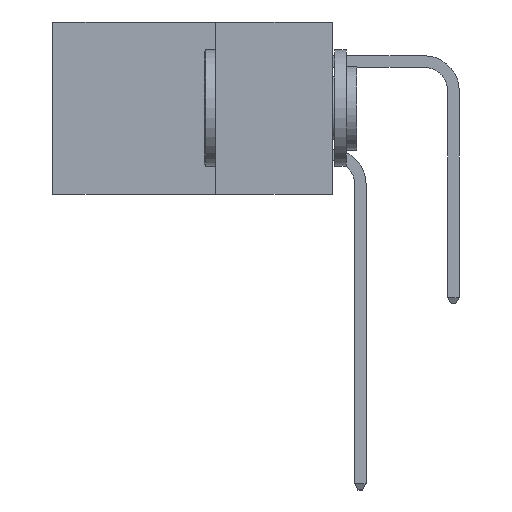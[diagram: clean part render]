
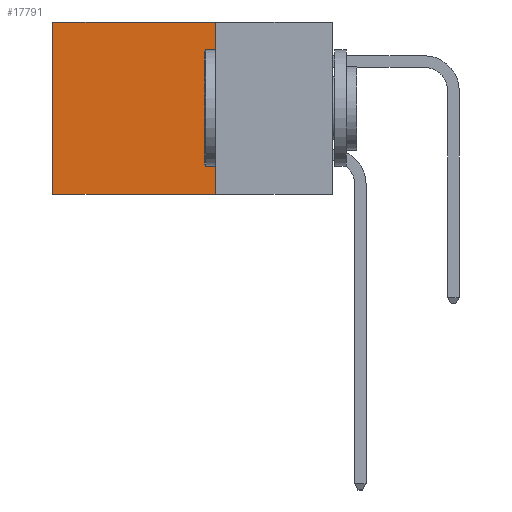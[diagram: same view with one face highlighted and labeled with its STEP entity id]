
A CAD part, left-side view. The second image highlights one B-rep face of the part: STEP entity #17791.
In plain terms, the highlighted planar face has unit normal (-1, 0, 0).
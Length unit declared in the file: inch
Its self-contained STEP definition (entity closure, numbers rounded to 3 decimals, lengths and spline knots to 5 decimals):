
#78 = EDGE_CURVE ( 'NONE', #25785, #3793, #5876, .T. ) ;
#630 = ORIENTED_EDGE ( 'NONE', *, *, #948, .F. ) ;
#640 = CARTESIAN_POINT ( 'NONE',  ( 0.2615, 0.25, -0.37 ) ) ;
#733 = DIRECTION ( 'NONE',  ( 0., 0., -1. ) ) ;
#948 = EDGE_CURVE ( 'NONE', #25785, #17775, #1451, .T. ) ;
#969 = CARTESIAN_POINT ( 'NONE',  ( 0.2615, 0.6, 0. ) ) ;
#1451 = LINE ( 'NONE', #21798, #7230 ) ;
#2162 = VERTEX_POINT ( 'NONE', #17096 ) ;
#3793 = VERTEX_POINT ( 'NONE', #969 ) ;
#5876 = LINE ( 'NONE', #25469, #10889 ) ;
#6764 = EDGE_CURVE ( 'NONE', #17775, #2162, #26233, .T. ) ;
#7230 = VECTOR ( 'NONE', #18867, 39.37008 ) ;
#8569 = EDGE_LOOP ( 'NONE', ( #27590, #21022, #630, #22609 ) ) ;
#9341 = PLANE ( 'NONE',  #25838 ) ;
#10278 = FACE_OUTER_BOUND ( 'NONE', #8569, .T. ) ;
#10849 = DIRECTION ( 'NONE',  ( 0., 1., 0. ) ) ;
#10889 = VECTOR ( 'NONE', #15597, 39.37008 ) ;
#13585 = DIRECTION ( 'NONE',  ( 1., 0., 0. ) ) ;
#14893 = VECTOR ( 'NONE', #10849, 39.37008 ) ;
#15597 = DIRECTION ( 'NONE',  ( 0., 1., 0. ) ) ;
#15653 = DIRECTION ( 'NONE',  ( 0., 0., -1. ) ) ;
#15832 = CARTESIAN_POINT ( 'NONE',  ( 0.2615, 0.25, 0. ) ) ;
#17096 = CARTESIAN_POINT ( 'NONE',  ( 0.2615, 0.6, -0.37 ) ) ;
#17204 = CARTESIAN_POINT ( 'NONE',  ( 0.2615, 0.25, -0.37 ) ) ;
#17261 = VECTOR ( 'NONE', #15653, 39.37008 ) ;
#17706 = CARTESIAN_POINT ( 'NONE',  ( 0.2615, 0.6, -0.37 ) ) ;
#17775 = VERTEX_POINT ( 'NONE', #19484 ) ;
#17791 = ADVANCED_FACE ( 'NONE', ( #10278 ), #9341, .F. ) ;
#18867 = DIRECTION ( 'NONE',  ( 0., 0., -1. ) ) ;
#19484 = CARTESIAN_POINT ( 'NONE',  ( 0.2615, 0.25, -0.37 ) ) ;
#21022 = ORIENTED_EDGE ( 'NONE', *, *, #6764, .F. ) ;
#21798 = CARTESIAN_POINT ( 'NONE',  ( 0.2615, 0.25, -0.37 ) ) ;
#22609 = ORIENTED_EDGE ( 'NONE', *, *, #78, .T. ) ;
#22681 = EDGE_CURVE ( 'NONE', #3793, #2162, #22941, .T. ) ;
#22941 = LINE ( 'NONE', #17706, #17261 ) ;
#25469 = CARTESIAN_POINT ( 'NONE',  ( 0.2615, 0.25, 0. ) ) ;
#25785 = VERTEX_POINT ( 'NONE', #15832 ) ;
#25838 = AXIS2_PLACEMENT_3D ( 'NONE', #640, #13585, #733 ) ;
#26233 = LINE ( 'NONE', #17204, #14893 ) ;
#27590 = ORIENTED_EDGE ( 'NONE', *, *, #22681, .T. ) ;
